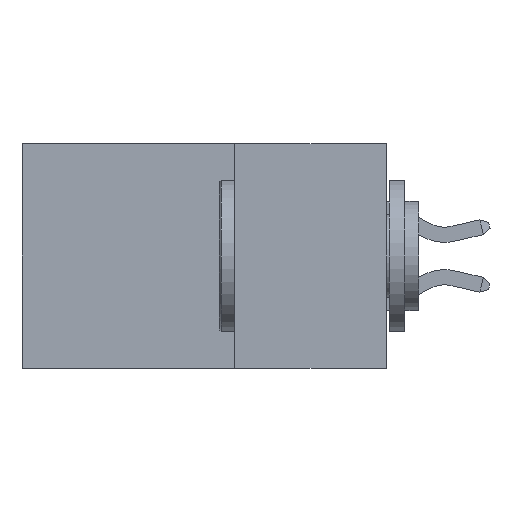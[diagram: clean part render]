
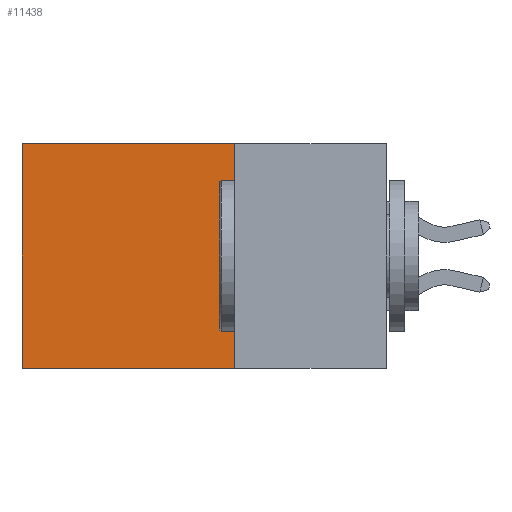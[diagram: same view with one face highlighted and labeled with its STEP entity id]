
A CAD part, left-side view. The second image highlights one B-rep face of the part: STEP entity #11438.
In plain terms, the highlighted planar face has unit normal (-1, 0, 0).
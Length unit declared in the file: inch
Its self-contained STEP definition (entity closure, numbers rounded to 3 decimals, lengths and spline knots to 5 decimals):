
#110 = ORIENTED_EDGE ( 'NONE', *, *, #17645, .F. ) ;
#2006 = DIRECTION ( 'NONE',  ( 0., 0., -1. ) ) ;
#2457 = DIRECTION ( 'NONE',  ( 0., 0., -1. ) ) ;
#2535 = LINE ( 'NONE', #2998, #16289 ) ;
#2738 = CARTESIAN_POINT ( 'NONE',  ( 0.298, 0.6, 0. ) ) ;
#2998 = CARTESIAN_POINT ( 'NONE',  ( 0.298, 0.25, -0.37 ) ) ;
#3223 = EDGE_CURVE ( 'NONE', #22723, #4421, #15997, .T. ) ;
#3679 = LINE ( 'NONE', #2738, #4821 ) ;
#4421 = VERTEX_POINT ( 'NONE', #21681 ) ;
#4821 = VECTOR ( 'NONE', #15300, 39.37008 ) ;
#7847 = LINE ( 'NONE', #13210, #16822 ) ;
#8503 = AXIS2_PLACEMENT_3D ( 'NONE', #9161, #12752, #2006 ) ;
#9161 = CARTESIAN_POINT ( 'NONE',  ( 0.298, 0.25, 0. ) ) ;
#10222 = DIRECTION ( 'NONE',  ( 0., 1., 0. ) ) ;
#11223 = VECTOR ( 'NONE', #16597, 39.37008 ) ;
#11370 = ORIENTED_EDGE ( 'NONE', *, *, #17908, .F. ) ;
#11438 = ADVANCED_FACE ( 'NONE', ( #20929 ), #18065, .F. ) ;
#12292 = CARTESIAN_POINT ( 'NONE',  ( 0.298, 0.6, -0.37 ) ) ;
#12416 = ORIENTED_EDGE ( 'NONE', *, *, #16715, .T. ) ;
#12752 = DIRECTION ( 'NONE',  ( 1., 0., 0. ) ) ;
#13210 = CARTESIAN_POINT ( 'NONE',  ( 0.298, 0.25, 0. ) ) ;
#15300 = DIRECTION ( 'NONE',  ( 0., 0., -1. ) ) ;
#15997 = LINE ( 'NONE', #16546, #11223 ) ;
#16289 = VECTOR ( 'NONE', #10222, 39.37008 ) ;
#16546 = CARTESIAN_POINT ( 'NONE',  ( 0.298, 0.25, 0. ) ) ;
#16597 = DIRECTION ( 'NONE',  ( 0., 1., 0. ) ) ;
#16715 = EDGE_CURVE ( 'NONE', #4421, #22734, #3679, .T. ) ;
#16822 = VECTOR ( 'NONE', #2457, 39.37008 ) ;
#17645 = EDGE_CURVE ( 'NONE', #22723, #18430, #7847, .T. ) ;
#17908 = EDGE_CURVE ( 'NONE', #18430, #22734, #2535, .T. ) ;
#18065 = PLANE ( 'NONE',  #8503 ) ;
#18430 = VERTEX_POINT ( 'NONE', #20572 ) ;
#19027 = EDGE_LOOP ( 'NONE', ( #12416, #11370, #110, #22165 ) ) ;
#20572 = CARTESIAN_POINT ( 'NONE',  ( 0.298, 0.25, -0.37 ) ) ;
#20929 = FACE_OUTER_BOUND ( 'NONE', #19027, .T. ) ;
#21681 = CARTESIAN_POINT ( 'NONE',  ( 0.298, 0.6, 0. ) ) ;
#22165 = ORIENTED_EDGE ( 'NONE', *, *, #3223, .T. ) ;
#22723 = VERTEX_POINT ( 'NONE', #22902 ) ;
#22734 = VERTEX_POINT ( 'NONE', #12292 ) ;
#22902 = CARTESIAN_POINT ( 'NONE',  ( 0.298, 0.25, 0. ) ) ;
